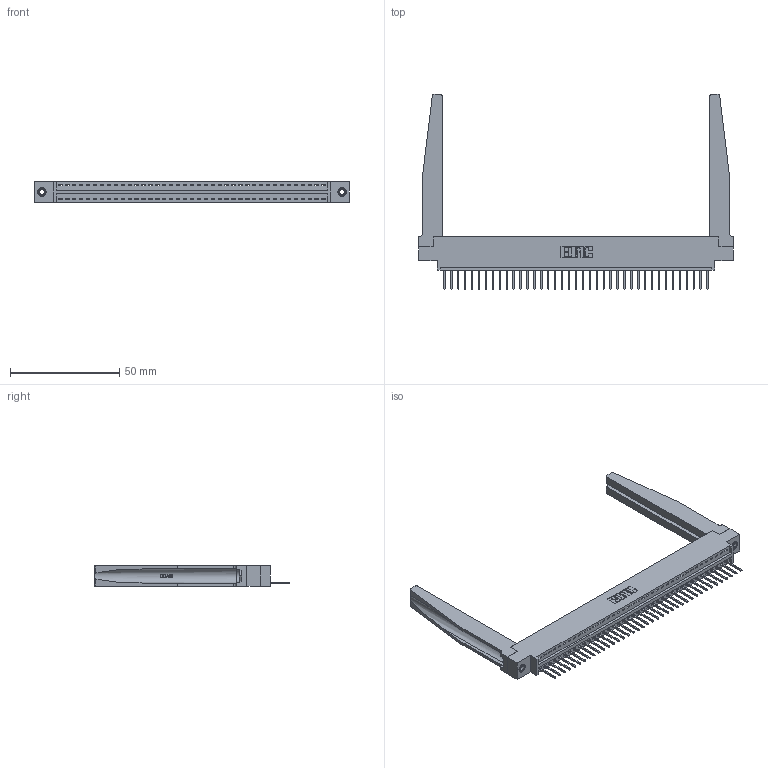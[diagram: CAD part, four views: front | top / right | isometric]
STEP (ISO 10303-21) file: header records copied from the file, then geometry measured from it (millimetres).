
FILE_DESCRIPTION (( 'STEP AP203' ), '1' );
FILE_NAME ('396-039-526-678.STEP', '2019-10-27T19:21:45', ( '' ), ( '' ), 'SwSTEP 2.0', 'SolidWorks 2016', '' );
FILE_SCHEMA (( 'CONFIG_CONTROL_DESIGN' ));
Length unit declared in the file: inch
Products named in the file (5): 346-220-078_345-220-078; 345-292-001_345-293-126; 346 Part_0.170 Offset - 0.156 Dia-TH; 396-039-526-678; 345-250-001_345-250-001-102
Assembly tree (44 placements, depth 2):
  396-039-526-678
    346 Part_0.170 Offset - 0.156 Dia-TH
    345-292-001_345-293-126  x39
    346-220-078_345-220-078  x2
    345-250-001_345-250-001-102  x2
Bounding box: 144.4 x 89.41 x 9.4 mm (x, y, z)
Volume: 20524.7 mm3; surface area: 23648.1 mm2
Topology: 44 solids, 44 shells, 2622 faces, 7813 edges, 5146 vertices
Faces by surface type: plane 1782, cylinder 788, bspline 36, cone 12, torus 4
Entity records: 29506 total; most frequent: CARTESIAN_POINT 5972, ORIENTED_EDGE 4834, DIRECTION 4257, EDGE_CURVE 2417, LINE 2035, VECTOR 2035, VERTEX_POINT 1604, AXIS2_PLACEMENT_3D 1111
